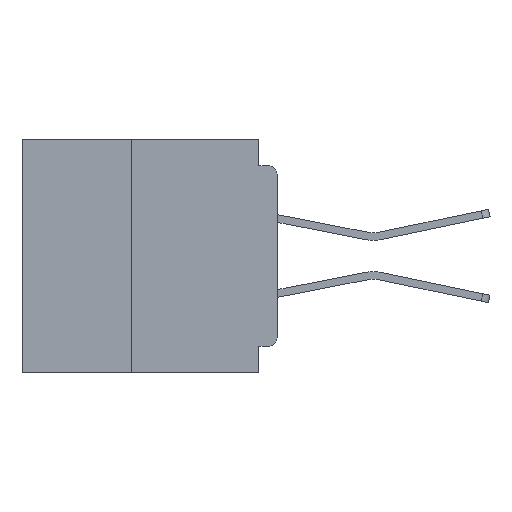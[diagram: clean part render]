
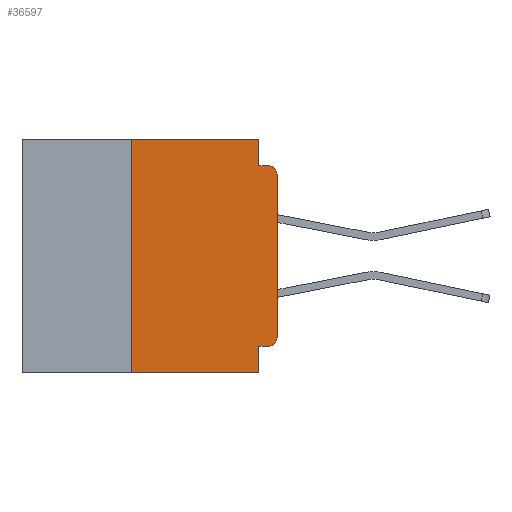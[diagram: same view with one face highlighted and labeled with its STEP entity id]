
A CAD part, left-side view. The second image highlights one B-rep face of the part: STEP entity #36597.
In plain terms, the highlighted planar face has unit normal (-1, 0, 0).
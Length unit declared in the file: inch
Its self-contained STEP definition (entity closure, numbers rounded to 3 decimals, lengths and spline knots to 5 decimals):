
#25 = DIRECTION ( 'NONE',  ( 0., 0., 1. ) ) ;
#104 = VECTOR ( 'NONE', #25, 39.37008 ) ;
#962 = ORIENTED_EDGE ( 'NONE', *, *, #4425, .F. ) ;
#1405 = EDGE_LOOP ( 'NONE', ( #29973, #39042, #20596, #31550, #33098, #962, #33397, #38291, #4059, #28841 ) ) ;
#2033 = VERTEX_POINT ( 'NONE', #8973 ) ;
#2114 = CARTESIAN_POINT ( 'NONE',  ( 0., 0.437, 0. ) ) ;
#2140 = CARTESIAN_POINT ( 'NONE',  ( 0., 0.25, -0.4 ) ) ;
#2700 = EDGE_CURVE ( 'NONE', #39125, #24363, #8990, .T. ) ;
#4059 = ORIENTED_EDGE ( 'NONE', *, *, #24561, .F. ) ;
#4264 = VECTOR ( 'NONE', #41736, 39.37008 ) ;
#4266 = DIRECTION ( 'NONE',  ( 0., 0., 1. ) ) ;
#4425 = EDGE_CURVE ( 'NONE', #46266, #2033, #11199, .T. ) ;
#5238 = VERTEX_POINT ( 'NONE', #24059 ) ;
#6067 = VECTOR ( 'NONE', #47384, 39.37008 ) ;
#6419 = VERTEX_POINT ( 'NONE', #30214 ) ;
#7240 = LINE ( 'NONE', #43745, #6067 ) ;
#8973 = CARTESIAN_POINT ( 'NONE',  ( 0., 0.25, 0. ) ) ;
#8990 = LINE ( 'NONE', #28234, #29911 ) ;
#9344 = LINE ( 'NONE', #41256, #27947 ) ;
#9810 = EDGE_CURVE ( 'NONE', #46266, #18131, #43218, .T. ) ;
#10506 = CARTESIAN_POINT ( 'NONE',  ( 0., 0.25, -0.4 ) ) ;
#10701 = VERTEX_POINT ( 'NONE', #31507 ) ;
#11199 = LINE ( 'NONE', #2140, #104 ) ;
#11864 = DIRECTION ( 'NONE',  ( 0., -1., 0. ) ) ;
#13268 = CARTESIAN_POINT ( 'NONE',  ( 0., 0.031, -0.045 ) ) ;
#13395 = DIRECTION ( 'NONE',  ( 0., 0., -1. ) ) ;
#16151 = CIRCLE ( 'NONE', #43973, 0.015 ) ;
#17853 = DIRECTION ( 'NONE',  ( -1., 0., 0. ) ) ;
#18131 = VERTEX_POINT ( 'NONE', #42833 ) ;
#18253 = CARTESIAN_POINT ( 'NONE',  ( 0., 0.015, -0.34 ) ) ;
#18480 = CARTESIAN_POINT ( 'NONE',  ( 0., 0., -0.045 ) ) ;
#19757 = EDGE_CURVE ( 'NONE', #5238, #18131, #27560, .T. ) ;
#19846 = CARTESIAN_POINT ( 'NONE',  ( 0., 0.031, -0.4 ) ) ;
#20596 = ORIENTED_EDGE ( 'NONE', *, *, #33827, .F. ) ;
#20786 = CARTESIAN_POINT ( 'NONE',  ( 0., 0., -0.34 ) ) ;
#21984 = DIRECTION ( 'NONE',  ( 0., 0., -1. ) ) ;
#24059 = CARTESIAN_POINT ( 'NONE',  ( 0., 0.031, -0.355 ) ) ;
#24089 = EDGE_CURVE ( 'NONE', #25663, #35347, #25435, .T. ) ;
#24263 = VECTOR ( 'NONE', #4266, 39.37008 ) ;
#24363 = VERTEX_POINT ( 'NONE', #13268 ) ;
#24561 = EDGE_CURVE ( 'NONE', #6419, #5238, #7240, .T. ) ;
#25435 = LINE ( 'NONE', #33901, #24263 ) ;
#25663 = VERTEX_POINT ( 'NONE', #20786 ) ;
#25793 = EDGE_CURVE ( 'NONE', #35347, #10701, #41146, .T. ) ;
#27560 = LINE ( 'NONE', #19846, #4264 ) ;
#27947 = VECTOR ( 'NONE', #11864, 39.37008 ) ;
#28186 = DIRECTION ( 'NONE',  ( 0., 0., -1. ) ) ;
#28234 = CARTESIAN_POINT ( 'NONE',  ( 0., 0.031, 0. ) ) ;
#28841 = ORIENTED_EDGE ( 'NONE', *, *, #41919, .T. ) ;
#29911 = VECTOR ( 'NONE', #28186, 39.37008 ) ;
#29973 = ORIENTED_EDGE ( 'NONE', *, *, #24089, .T. ) ;
#30114 = AXIS2_PLACEMENT_3D ( 'NONE', #2114, #35407, #13395 ) ;
#30214 = CARTESIAN_POINT ( 'NONE',  ( 0., 0.015, -0.355 ) ) ;
#31393 = AXIS2_PLACEMENT_3D ( 'NONE', #39789, #17853, #43480 ) ;
#31507 = CARTESIAN_POINT ( 'NONE',  ( 0., 0.015, -0.045 ) ) ;
#31550 = ORIENTED_EDGE ( 'NONE', *, *, #2700, .F. ) ;
#31824 = VECTOR ( 'NONE', #40560, 39.37008 ) ;
#32756 = FACE_OUTER_BOUND ( 'NONE', #1405, .T. ) ;
#33098 = ORIENTED_EDGE ( 'NONE', *, *, #42679, .F. ) ;
#33397 = ORIENTED_EDGE ( 'NONE', *, *, #9810, .T. ) ;
#33538 = VECTOR ( 'NONE', #40777, 39.37008 ) ;
#33827 = EDGE_CURVE ( 'NONE', #24363, #10701, #42626, .T. ) ;
#33901 = CARTESIAN_POINT ( 'NONE',  ( 0., 0., 0. ) ) ;
#35347 = VERTEX_POINT ( 'NONE', #42866 ) ;
#35407 = DIRECTION ( 'NONE',  ( 1., 0., 0. ) ) ;
#36597 = ADVANCED_FACE ( 'NONE', ( #32756 ), #46269, .F. ) ;
#37090 = CARTESIAN_POINT ( 'NONE',  ( 0., 0.031, 0. ) ) ;
#37119 = CARTESIAN_POINT ( 'NONE',  ( 0., 0.437, -0.4 ) ) ;
#38291 = ORIENTED_EDGE ( 'NONE', *, *, #19757, .F. ) ;
#39042 = ORIENTED_EDGE ( 'NONE', *, *, #25793, .T. ) ;
#39125 = VERTEX_POINT ( 'NONE', #37090 ) ;
#39789 = CARTESIAN_POINT ( 'NONE',  ( 0., 0.015, -0.06 ) ) ;
#40560 = DIRECTION ( 'NONE',  ( 0., -1., 0. ) ) ;
#40777 = DIRECTION ( 'NONE',  ( 0., -1., 0. ) ) ;
#41146 = CIRCLE ( 'NONE', #31393, 0.015 ) ;
#41256 = CARTESIAN_POINT ( 'NONE',  ( 0., 0.437, 0. ) ) ;
#41736 = DIRECTION ( 'NONE',  ( 0., 0., -1. ) ) ;
#41919 = EDGE_CURVE ( 'NONE', #6419, #25663, #16151, .T. ) ;
#42626 = LINE ( 'NONE', #18480, #31824 ) ;
#42679 = EDGE_CURVE ( 'NONE', #2033, #39125, #9344, .T. ) ;
#42833 = CARTESIAN_POINT ( 'NONE',  ( 0., 0.031, -0.4 ) ) ;
#42866 = CARTESIAN_POINT ( 'NONE',  ( 0., 0., -0.06 ) ) ;
#43218 = LINE ( 'NONE', #37119, #33538 ) ;
#43480 = DIRECTION ( 'NONE',  ( 0., 0., -1. ) ) ;
#43745 = CARTESIAN_POINT ( 'NONE',  ( 0., 0., -0.355 ) ) ;
#43880 = DIRECTION ( 'NONE',  ( -1., 0., 0. ) ) ;
#43973 = AXIS2_PLACEMENT_3D ( 'NONE', #18253, #43880, #21984 ) ;
#46266 = VERTEX_POINT ( 'NONE', #10506 ) ;
#46269 = PLANE ( 'NONE',  #30114 ) ;
#47384 = DIRECTION ( 'NONE',  ( 0., 1., 0. ) ) ;
